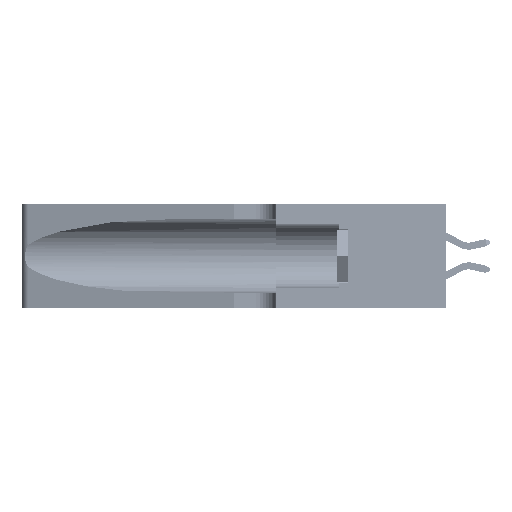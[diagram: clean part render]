
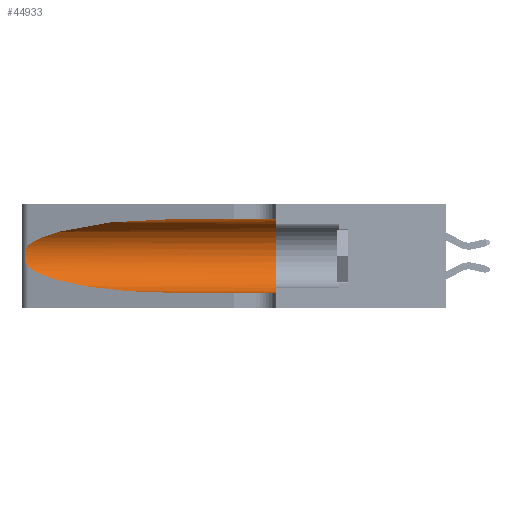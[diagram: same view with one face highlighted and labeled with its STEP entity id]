
A CAD part, left-side view. The second image highlights one B-rep face of the part: STEP entity #44933.
In plain terms, the highlighted cylindrical face has radius 3.308 mm (diameter 6.617 mm), a partial arc.
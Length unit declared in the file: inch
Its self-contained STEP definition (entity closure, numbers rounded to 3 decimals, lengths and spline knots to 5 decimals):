
#31 = CARTESIAN_POINT ( 'NONE',  ( 0.2373, 1.15595, 0.28018 ) ) ;
#1258 = DIRECTION ( 'NONE',  ( 0., 0., 1. ) ) ;
#1928 = AXIS2_PLACEMENT_3D ( 'NONE', #45400, #23581, #1258 ) ;
#3524 = CARTESIAN_POINT ( 'NONE',  ( 0.26017, 1.23833, 0.17102 ) ) ;
#4262 = ORIENTED_EDGE ( 'NONE', *, *, #27703, .T. ) ;
#4400 = CARTESIAN_POINT ( 'NONE',  ( 0.1305, 0.35, 0.31525 ) ) ;
#4525 = CARTESIAN_POINT ( 'NONE',  ( 0.18966, 0.96281, 0.05475 ) ) ;
#6765 = EDGE_CURVE ( 'NONE', #32416, #9792, #25573, .T. ) ;
#6771 = ORIENTED_EDGE ( 'NONE', *, *, #22969, .T. ) ;
#6904 = CARTESIAN_POINT ( 'NONE',  ( 0.1305, 1.61858, 0.05475 ) ) ;
#7098 = CARTESIAN_POINT ( 'NONE',  ( 0.25487, 1.22718, 0.22369 ) ) ;
#7251 = CARTESIAN_POINT ( 'NONE',  ( 0.25789, 1.23486, 0.15765 ) ) ;
#8229 = DIRECTION ( 'NONE',  ( 0., -1., 0. ) ) ;
#9047 = ORIENTED_EDGE ( 'NONE', *, *, #17217, .F. ) ;
#9792 = VERTEX_POINT ( 'NONE', #21425 ) ;
#11032 = CARTESIAN_POINT ( 'NONE',  ( 0.25555, 1.22993, 0.14849 ) ) ;
#12026 = AXIS2_PLACEMENT_3D ( 'NONE', #15783, #8229, #41388 ) ;
#13152 = EDGE_LOOP ( 'NONE', ( #6771, #16827, #4262, #17651, #29224, #9047 ) ) ;
#14924 = CARTESIAN_POINT ( 'NONE',  ( 0.1305, 0.72297, 0.31525 ) ) ;
#15783 = CARTESIAN_POINT ( 'NONE',  ( 0.1305, 1.61858, 0.185 ) ) ;
#16449 = CARTESIAN_POINT ( 'NONE',  ( 0.1305, 0.72297, 0.31525 ) ) ;
#16827 = ORIENTED_EDGE ( 'NONE', *, *, #34350, .T. ) ;
#17217 = EDGE_CURVE ( 'NONE', #29761, #17408, #17748, .T. ) ;
#17408 = VERTEX_POINT ( 'NONE', #4400 ) ;
#17640 = DIRECTION ( 'NONE',  ( 0., -1., 0. ) ) ;
#17651 = ORIENTED_EDGE ( 'NONE', *, *, #6765, .T. ) ;
#17748 = LINE ( 'NONE', #32204, #26370 ) ;
#18372 = CARTESIAN_POINT ( 'NONE',  ( 0.25787, 1.23484, 0.2124 ) ) ;
#21425 = CARTESIAN_POINT ( 'NONE',  ( 0.1305, 0.35, 0.05475 ) ) ;
#22093 = CARTESIAN_POINT ( 'NONE',  ( 0.26018, 1.23835, 0.19895 ) ) ;
#22489 = CIRCLE ( 'NONE', #1928, 0.13025 ) ;
#22969 = EDGE_CURVE ( 'NONE', #29761, #33066, #34381, .T. ) ;
#23079 = CARTESIAN_POINT ( 'NONE',  ( 0.2373, 1.15595, 0.08982 ) ) ;
#23581 = DIRECTION ( 'NONE',  ( 0., 1., 0. ) ) ;
#24456 = CYLINDRICAL_SURFACE ( 'NONE', #12026, 0.13025 ) ;
#25573 = LINE ( 'NONE', #6904, #42663 ) ;
#25775 = CARTESIAN_POINT ( 'NONE',  ( 0.26075, 1.23896, 0.178 ) ) ;
#25940 = VERTEX_POINT ( 'NONE', #26745 ) ;
#26034 = CARTESIAN_POINT ( 'NONE',  ( 0.25487, 1.22718, 0.22369 ) ) ;
#26370 = VECTOR ( 'NONE', #17640, 39.37008 ) ;
#26745 = CARTESIAN_POINT ( 'NONE',  ( 0.25487, 1.22718, 0.14631 ) ) ;
#27703 = EDGE_CURVE ( 'NONE', #25940, #32416, #37295, .T. ) ;
#28858 = B_SPLINE_CURVE_WITH_KNOTS ( 'NONE', 3,
 ( #7098, #36585, #40258, #18372, #43935, #22093, #47593, #25775, #3524, #29429, #7251, #33065, #11032, #36728 ),
 .UNSPECIFIED., .F., .F.,
 ( 4, 2, 2, 2, 2, 2, 4 ),
 ( 0., 0.00027, 0.00053, 0.00107, 0.0016, 0.00187, 0.00214 ),
 .UNSPECIFIED. ) ;
#29075 = DIRECTION ( 'NONE',  ( 0., -1., 0. ) ) ;
#29224 = ORIENTED_EDGE ( 'NONE', *, *, #35787, .F. ) ;
#29429 = CARTESIAN_POINT ( 'NONE',  ( 0.25856, 1.23593, 0.16098 ) ) ;
#29761 = VERTEX_POINT ( 'NONE', #16449 ) ;
#30407 = CARTESIAN_POINT ( 'NONE',  ( 0.1305, 0.72297, 0.05475 ) ) ;
#32204 = CARTESIAN_POINT ( 'NONE',  ( 0.1305, 1.61858, 0.31525 ) ) ;
#32416 = VERTEX_POINT ( 'NONE', #47457 ) ;
#33065 = CARTESIAN_POINT ( 'NONE',  ( 0.25639, 1.23186, 0.15144 ) ) ;
#33066 = VERTEX_POINT ( 'NONE', #44375 ) ;
#34350 = EDGE_CURVE ( 'NONE', #33066, #25940, #28858, .T. ) ;
#34381 =( BOUNDED_CURVE ( )  B_SPLINE_CURVE ( 3, ( #14924, #44204, #31, #26034 ),
 .UNSPECIFIED., .F., .F. ) 
 B_SPLINE_CURVE_WITH_KNOTS ( ( 4, 4 ),
 ( 1.5708, 2.84003 ),
 .UNSPECIFIED. ) 
 CURVE ( )  GEOMETRIC_REPRESENTATION_ITEM ( )  RATIONAL_B_SPLINE_CURVE ( ( 1., 0.87, 0.87, 1. ) ) 
 REPRESENTATION_ITEM ( '' )  );
#35787 = EDGE_CURVE ( 'NONE', #17408, #9792, #22489, .T. ) ;
#36585 = CARTESIAN_POINT ( 'NONE',  ( 0.25555, 1.22994, 0.2215 ) ) ;
#36728 = CARTESIAN_POINT ( 'NONE',  ( 0.25487, 1.22718, 0.14631 ) ) ;
#37295 =( BOUNDED_CURVE ( )  B_SPLINE_CURVE ( 3, ( #41248, #23079, #4525, #30407 ),
 .UNSPECIFIED., .F., .F. ) 
 B_SPLINE_CURVE_WITH_KNOTS ( ( 4, 4 ),
 ( 3.44316, 4.71239 ),
 .UNSPECIFIED. ) 
 CURVE ( )  GEOMETRIC_REPRESENTATION_ITEM ( )  RATIONAL_B_SPLINE_CURVE ( ( 1., 0.87, 0.87, 1. ) ) 
 REPRESENTATION_ITEM ( '' )  );
#40258 = CARTESIAN_POINT ( 'NONE',  ( 0.25639, 1.23184, 0.21858 ) ) ;
#41248 = CARTESIAN_POINT ( 'NONE',  ( 0.25487, 1.22718, 0.14631 ) ) ;
#41388 = DIRECTION ( 'NONE',  ( 0., 0., -1. ) ) ;
#42663 = VECTOR ( 'NONE', #29075, 39.37008 ) ;
#43832 = FACE_OUTER_BOUND ( 'NONE', #13152, .T. ) ;
#43935 = CARTESIAN_POINT ( 'NONE',  ( 0.25854, 1.2359, 0.20912 ) ) ;
#44204 = CARTESIAN_POINT ( 'NONE',  ( 0.18966, 0.96281, 0.31525 ) ) ;
#44375 = CARTESIAN_POINT ( 'NONE',  ( 0.25487, 1.22718, 0.22369 ) ) ;
#44933 = ADVANCED_FACE ( 'NONE', ( #43832 ), #24456, .F. ) ;
#45400 = CARTESIAN_POINT ( 'NONE',  ( 0.1305, 0.35, 0.185 ) ) ;
#47457 = CARTESIAN_POINT ( 'NONE',  ( 0.1305, 0.72297, 0.05475 ) ) ;
#47593 = CARTESIAN_POINT ( 'NONE',  ( 0.26075, 1.23896, 0.19203 ) ) ;
